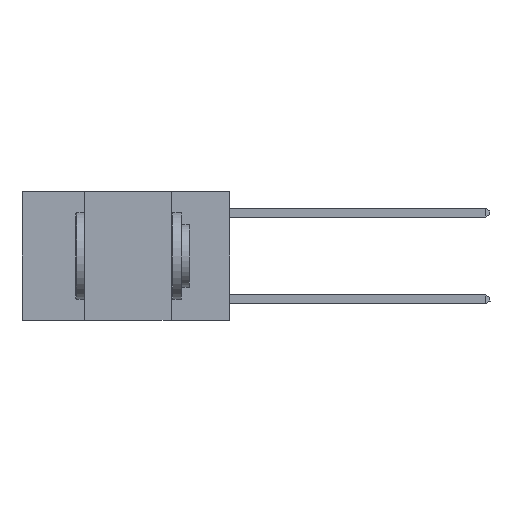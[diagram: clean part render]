
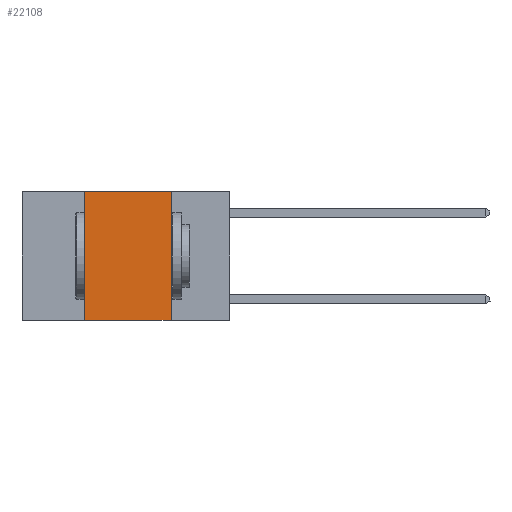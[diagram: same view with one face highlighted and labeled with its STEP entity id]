
A CAD part, left-side view. The second image highlights one B-rep face of the part: STEP entity #22108.
In plain terms, the highlighted planar face has unit normal (-1, 0, 0).
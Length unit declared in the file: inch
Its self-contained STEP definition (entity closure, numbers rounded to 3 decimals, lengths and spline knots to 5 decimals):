
#176 = CARTESIAN_POINT ( 'NONE',  ( 0., 0.42, 0. ) ) ;
#458 = VERTEX_POINT ( 'NONE', #9081 ) ;
#1021 = VECTOR ( 'NONE', #18481, 39.37008 ) ;
#1823 = VECTOR ( 'NONE', #14317, 39.37008 ) ;
#2262 = EDGE_CURVE ( 'NONE', #27114, #15022, #25022, .T. ) ;
#2394 = CARTESIAN_POINT ( 'NONE',  ( 0., 0.17, -0.37 ) ) ;
#4309 = FACE_OUTER_BOUND ( 'NONE', #7573, .T. ) ;
#5305 = PLANE ( 'NONE',  #16633 ) ;
#5495 = CARTESIAN_POINT ( 'NONE',  ( 0., 0.17, 0. ) ) ;
#5525 = CARTESIAN_POINT ( 'NONE',  ( 0., 0.42, -0.37 ) ) ;
#6036 = LINE ( 'NONE', #176, #27180 ) ;
#7526 = DIRECTION ( 'NONE',  ( 1., 0., 0. ) ) ;
#7573 = EDGE_LOOP ( 'NONE', ( #25490, #8800, #21104, #16000 ) ) ;
#7976 = CARTESIAN_POINT ( 'NONE',  ( 0., 0.17, 0. ) ) ;
#8800 = ORIENTED_EDGE ( 'NONE', *, *, #25699, .F. ) ;
#9081 = CARTESIAN_POINT ( 'NONE',  ( 0., 0.42, 0. ) ) ;
#12717 = LINE ( 'NONE', #18288, #1021 ) ;
#14317 = DIRECTION ( 'NONE',  ( 0., 0., -1. ) ) ;
#15022 = VERTEX_POINT ( 'NONE', #2394 ) ;
#15370 = CARTESIAN_POINT ( 'NONE',  ( 0., 0.6, -0.37 ) ) ;
#15579 = LINE ( 'NONE', #15370, #26435 ) ;
#16000 = ORIENTED_EDGE ( 'NONE', *, *, #23298, .T. ) ;
#16633 = AXIS2_PLACEMENT_3D ( 'NONE', #18433, #7526, #22805 ) ;
#17564 = DIRECTION ( 'NONE',  ( 0., -1., 0. ) ) ;
#17701 = DIRECTION ( 'NONE',  ( 0., 0., 1. ) ) ;
#18288 = CARTESIAN_POINT ( 'NONE',  ( 0., 0.6, 0. ) ) ;
#18433 = CARTESIAN_POINT ( 'NONE',  ( 0., 0.6, 0. ) ) ;
#18481 = DIRECTION ( 'NONE',  ( 0., -1., 0. ) ) ;
#19569 = VERTEX_POINT ( 'NONE', #5525 ) ;
#21104 = ORIENTED_EDGE ( 'NONE', *, *, #21851, .F. ) ;
#21851 = EDGE_CURVE ( 'NONE', #19569, #458, #6036, .T. ) ;
#22108 = ADVANCED_FACE ( 'NONE', ( #4309 ), #5305, .F. ) ;
#22805 = DIRECTION ( 'NONE',  ( 0., 0., -1. ) ) ;
#23298 = EDGE_CURVE ( 'NONE', #19569, #15022, #15579, .T. ) ;
#25022 = LINE ( 'NONE', #7976, #1823 ) ;
#25490 = ORIENTED_EDGE ( 'NONE', *, *, #2262, .F. ) ;
#25699 = EDGE_CURVE ( 'NONE', #458, #27114, #12717, .T. ) ;
#26435 = VECTOR ( 'NONE', #17564, 39.37008 ) ;
#27114 = VERTEX_POINT ( 'NONE', #5495 ) ;
#27180 = VECTOR ( 'NONE', #17701, 39.37008 ) ;
